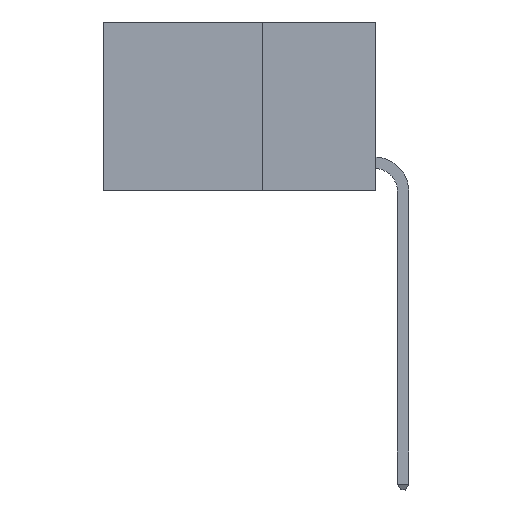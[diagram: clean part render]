
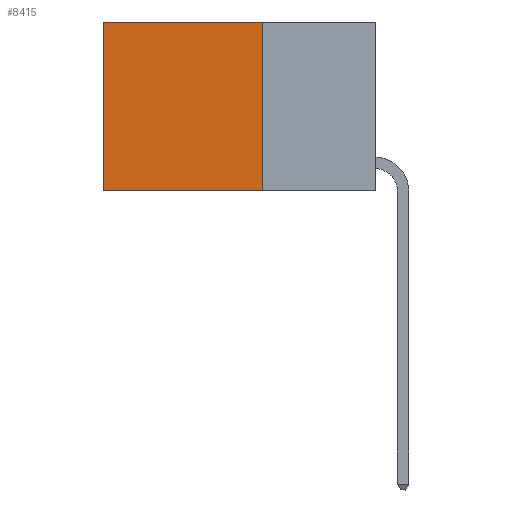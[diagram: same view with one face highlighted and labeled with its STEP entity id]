
A CAD part, left-side view. The second image highlights one B-rep face of the part: STEP entity #8415.
In plain terms, the highlighted planar face has unit normal (-1, 0, 0).
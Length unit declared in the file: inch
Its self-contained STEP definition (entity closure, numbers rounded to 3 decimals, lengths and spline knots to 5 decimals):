
#121 = EDGE_CURVE ( 'NONE', #276, #10595, #7574, .T. ) ;
#276 = VERTEX_POINT ( 'NONE', #10295 ) ;
#327 = DIRECTION ( 'NONE',  ( 0., 1., 0. ) ) ;
#689 = EDGE_CURVE ( 'NONE', #9985, #10595, #4674, .T. ) ;
#1148 = DIRECTION ( 'NONE',  ( 0., 1., 0. ) ) ;
#2266 = LINE ( 'NONE', #8378, #5496 ) ;
#2273 = ORIENTED_EDGE ( 'NONE', *, *, #11855, .F. ) ;
#4508 = VECTOR ( 'NONE', #327, 39.37008 ) ;
#4674 = LINE ( 'NONE', #8479, #4508 ) ;
#5496 = VECTOR ( 'NONE', #14768, 39.37008 ) ;
#5983 = PLANE ( 'NONE',  #8510 ) ;
#7137 = VERTEX_POINT ( 'NONE', #14974 ) ;
#7260 = DIRECTION ( 'NONE',  ( 0., 0., -1. ) ) ;
#7471 = VECTOR ( 'NONE', #9940, 39.37008 ) ;
#7574 = LINE ( 'NONE', #8300, #7471 ) ;
#7925 = CARTESIAN_POINT ( 'NONE',  ( 0.2625, 0.25, 0. ) ) ;
#8300 = CARTESIAN_POINT ( 'NONE',  ( 0.2625, 0.6, 0. ) ) ;
#8378 = CARTESIAN_POINT ( 'NONE',  ( 0.2625, 0.25, 0. ) ) ;
#8415 = ADVANCED_FACE ( 'NONE', ( #14097 ), #5983, .F. ) ;
#8479 = CARTESIAN_POINT ( 'NONE',  ( 0.2625, 0.25, -0.37 ) ) ;
#8510 = AXIS2_PLACEMENT_3D ( 'NONE', #9856, #14988, #7260 ) ;
#9186 = VECTOR ( 'NONE', #1148, 39.37008 ) ;
#9626 = ORIENTED_EDGE ( 'NONE', *, *, #121, .T. ) ;
#9688 = CARTESIAN_POINT ( 'NONE',  ( 0.2625, 0.25, -0.37 ) ) ;
#9856 = CARTESIAN_POINT ( 'NONE',  ( 0.2625, 0.25, 0. ) ) ;
#9940 = DIRECTION ( 'NONE',  ( 0., 0., -1. ) ) ;
#9985 = VERTEX_POINT ( 'NONE', #9688 ) ;
#9986 = ORIENTED_EDGE ( 'NONE', *, *, #689, .F. ) ;
#10295 = CARTESIAN_POINT ( 'NONE',  ( 0.2625, 0.6, 0. ) ) ;
#10595 = VERTEX_POINT ( 'NONE', #15858 ) ;
#11617 = EDGE_CURVE ( 'NONE', #7137, #276, #12632, .T. ) ;
#11855 = EDGE_CURVE ( 'NONE', #7137, #9985, #2266, .T. ) ;
#12632 = LINE ( 'NONE', #7925, #9186 ) ;
#13417 = EDGE_LOOP ( 'NONE', ( #9626, #9986, #2273, #16801 ) ) ;
#14097 = FACE_OUTER_BOUND ( 'NONE', #13417, .T. ) ;
#14768 = DIRECTION ( 'NONE',  ( 0., 0., -1. ) ) ;
#14974 = CARTESIAN_POINT ( 'NONE',  ( 0.2625, 0.25, 0. ) ) ;
#14988 = DIRECTION ( 'NONE',  ( 1., 0., 0. ) ) ;
#15858 = CARTESIAN_POINT ( 'NONE',  ( 0.2625, 0.6, -0.37 ) ) ;
#16801 = ORIENTED_EDGE ( 'NONE', *, *, #11617, .T. ) ;
